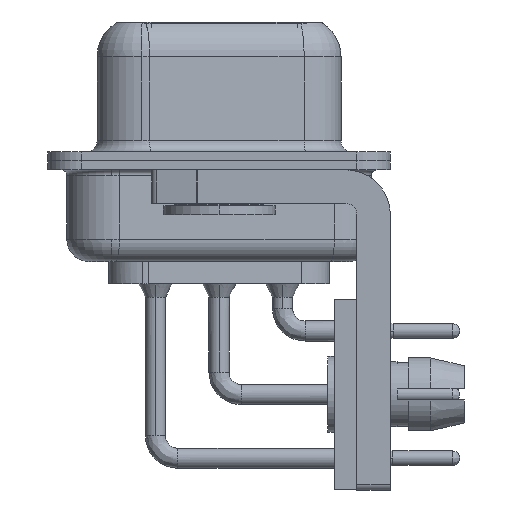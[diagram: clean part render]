
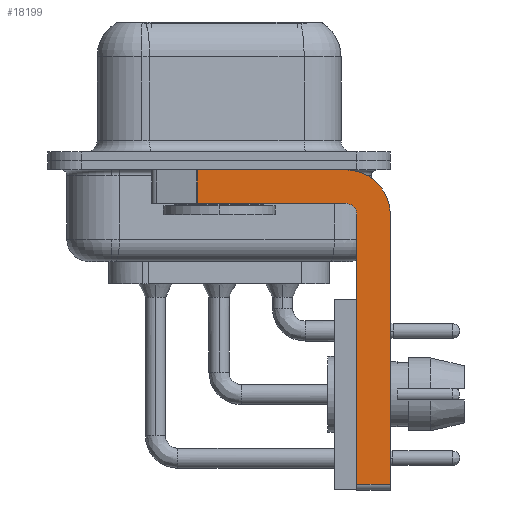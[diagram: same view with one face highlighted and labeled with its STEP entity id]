
A CAD part, left-side view. The second image highlights one B-rep face of the part: STEP entity #18199.
In plain terms, the highlighted planar face has unit normal (-1, 0, 0).
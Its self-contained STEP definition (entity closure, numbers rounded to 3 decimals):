
#27 = VERTEX_POINT ( 'NONE', #31115 ) ;
#559 = DIRECTION ( 'NONE',  ( 0., 0., -1. ) ) ;
#1104 = DIRECTION ( 'NONE',  ( 0., -1., 0. ) ) ;
#1156 = CIRCLE ( 'NONE', #36567, 2. ) ;
#1165 = ORIENTED_EDGE ( 'NONE', *, *, #1186, .F. ) ;
#1186 = EDGE_CURVE ( 'NONE', #9846, #27, #39095, .T. ) ;
#1559 = CARTESIAN_POINT ( 'NONE',  ( -2.9, 0.978, -0.4 ) ) ;
#1661 = EDGE_CURVE ( 'NONE', #2160, #18015, #1156, .T. ) ;
#1740 = CARTESIAN_POINT ( 'NONE',  ( -2.9, 0.978, -1.9 ) ) ;
#2160 = VERTEX_POINT ( 'NONE', #2224 ) ;
#2224 = CARTESIAN_POINT ( 'NONE',  ( -2.9, -5.65, -0.4 ) ) ;
#3940 = EDGE_CURVE ( 'NONE', #18015, #17202, #6827, .T. ) ;
#5509 = DIRECTION ( 'NONE',  ( 0., 1., 0. ) ) ;
#5706 = CARTESIAN_POINT ( 'NONE',  ( -2.9, -5.65, -2.4 ) ) ;
#6827 = LINE ( 'NONE', #18478, #14051 ) ;
#7092 = CARTESIAN_POINT ( 'NONE',  ( -2.9, -7.65, -14.45 ) ) ;
#8824 = DIRECTION ( 'NONE',  ( 0., 0., 1. ) ) ;
#9289 = CARTESIAN_POINT ( 'NONE',  ( -2.9, 0.978, -1.9 ) ) ;
#9846 = VERTEX_POINT ( 'NONE', #24684 ) ;
#10314 = ORIENTED_EDGE ( 'NONE', *, *, #39624, .F. ) ;
#10559 = CARTESIAN_POINT ( 'NONE',  ( -2.9, -5.65, -1.9 ) ) ;
#10843 = ORIENTED_EDGE ( 'NONE', *, *, #24672, .F. ) ;
#11042 = DIRECTION ( 'NONE',  ( 0., 0., -1. ) ) ;
#11713 = CARTESIAN_POINT ( 'NONE',  ( -2.9, -5.65, -1.9 ) ) ;
#14051 = VECTOR ( 'NONE', #18897, 1000. ) ;
#14298 = AXIS2_PLACEMENT_3D ( 'NONE', #5706, #27128, #8824 ) ;
#15582 = DIRECTION ( 'NONE',  ( 0., 0., -1. ) ) ;
#15671 = DIRECTION ( 'NONE',  ( 1., 0., 0. ) ) ;
#15726 = CARTESIAN_POINT ( 'NONE',  ( -2.9, -5.65, -2.4 ) ) ;
#16650 = ORIENTED_EDGE ( 'NONE', *, *, #1661, .F. ) ;
#16738 = EDGE_CURVE ( 'NONE', #31654, #23160, #34239, .T. ) ;
#17202 = VERTEX_POINT ( 'NONE', #7092 ) ;
#17869 = VECTOR ( 'NONE', #1104, 1000. ) ;
#18015 = VERTEX_POINT ( 'NONE', #39604 ) ;
#18199 = ADVANCED_FACE ( 'NONE', ( #38002 ), #37299, .F. ) ;
#18391 = ORIENTED_EDGE ( 'NONE', *, *, #24382, .F. ) ;
#18478 = CARTESIAN_POINT ( 'NONE',  ( -2.9, -7.65, -2.4 ) ) ;
#18897 = DIRECTION ( 'NONE',  ( 0., 0., -1. ) ) ;
#18953 = DIRECTION ( 'NONE',  ( 1., 0., 0. ) ) ;
#19220 = ORIENTED_EDGE ( 'NONE', *, *, #3940, .F. ) ;
#19661 = VERTEX_POINT ( 'NONE', #10559 ) ;
#19804 = LINE ( 'NONE', #34751, #17869 ) ;
#21412 = CIRCLE ( 'NONE', #14298, 0.5 ) ;
#22767 = VECTOR ( 'NONE', #26420, 1000. ) ;
#22977 = ORIENTED_EDGE ( 'NONE', *, *, #16738, .T. ) ;
#23160 = VERTEX_POINT ( 'NONE', #9289 ) ;
#23233 = AXIS2_PLACEMENT_3D ( 'NONE', #31131, #18953, #559 ) ;
#24382 = EDGE_CURVE ( 'NONE', #31654, #2160, #19804, .T. ) ;
#24544 = VECTOR ( 'NONE', #5509, 1000. ) ;
#24672 = EDGE_CURVE ( 'NONE', #19661, #23160, #27410, .T. ) ;
#24684 = CARTESIAN_POINT ( 'NONE',  ( -2.9, -6.15, -14.45 ) ) ;
#26063 = EDGE_CURVE ( 'NONE', #9846, #17202, #36408, .T. ) ;
#26420 = DIRECTION ( 'NONE',  ( 0., 0., 1. ) ) ;
#26723 = CARTESIAN_POINT ( 'NONE',  ( -2.9, -6.15, -14.7 ) ) ;
#27128 = DIRECTION ( 'NONE',  ( -1., 0., 0. ) ) ;
#27410 = LINE ( 'NONE', #11713, #24544 ) ;
#31115 = CARTESIAN_POINT ( 'NONE',  ( -2.9, -6.15, -2.4 ) ) ;
#31131 = CARTESIAN_POINT ( 'NONE',  ( -2.9, -5.65, -2.4 ) ) ;
#31654 = VERTEX_POINT ( 'NONE', #1559 ) ;
#33269 = VECTOR ( 'NONE', #11042, 1000. ) ;
#34239 = LINE ( 'NONE', #1740, #33269 ) ;
#34486 = CARTESIAN_POINT ( 'NONE',  ( -2.9, -5.65, -14.45 ) ) ;
#34751 = CARTESIAN_POINT ( 'NONE',  ( -2.9, 3., -0.4 ) ) ;
#34838 = EDGE_LOOP ( 'NONE', ( #18391, #22977, #10843, #10314, #1165, #35940, #19220, #16650 ) ) ;
#35440 = VECTOR ( 'NONE', #37582, 1000. ) ;
#35940 = ORIENTED_EDGE ( 'NONE', *, *, #26063, .T. ) ;
#36408 = LINE ( 'NONE', #34486, #35440 ) ;
#36567 = AXIS2_PLACEMENT_3D ( 'NONE', #15726, #15671, #15582 ) ;
#37299 = PLANE ( 'NONE',  #23233 ) ;
#37582 = DIRECTION ( 'NONE',  ( 0., -1., 0. ) ) ;
#38002 = FACE_OUTER_BOUND ( 'NONE', #34838, .T. ) ;
#39095 = LINE ( 'NONE', #26723, #22767 ) ;
#39604 = CARTESIAN_POINT ( 'NONE',  ( -2.9, -7.65, -2.4 ) ) ;
#39624 = EDGE_CURVE ( 'NONE', #27, #19661, #21412, .T. ) ;
